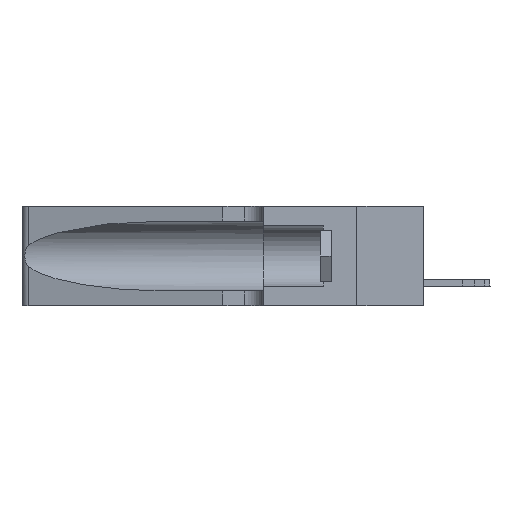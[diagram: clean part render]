
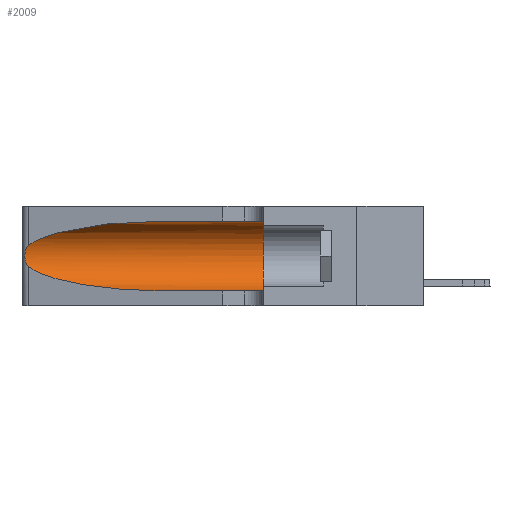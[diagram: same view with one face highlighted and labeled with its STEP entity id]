
A CAD part, left-side view. The second image highlights one B-rep face of the part: STEP entity #2009.
In plain terms, the highlighted cylindrical face has radius 3.308 mm (diameter 6.617 mm), a partial arc.
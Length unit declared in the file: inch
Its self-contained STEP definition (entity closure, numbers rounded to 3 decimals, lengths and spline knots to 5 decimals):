
#118 = VECTOR ( 'NONE', #12408, 39.37008 ) ;
#494 = CARTESIAN_POINT ( 'NONE',  ( 0.26075, 1.23896, 0.19203 ) ) ;
#770 = DIRECTION ( 'NONE',  ( 0., -1., 0. ) ) ;
#2009 = ADVANCED_FACE ( 'NONE', ( #16405 ), #30683, .F. ) ;
#2589 = CARTESIAN_POINT ( 'NONE',  ( 0.25856, 1.23593, 0.16098 ) ) ;
#2750 = CARTESIAN_POINT ( 'NONE',  ( 0.1305, 0.35, 0.31525 ) ) ;
#2858 = VERTEX_POINT ( 'NONE', #18748 ) ;
#3117 = DIRECTION ( 'NONE',  ( 0., 1., 0. ) ) ;
#3706 = EDGE_CURVE ( 'NONE', #29755, #21667, #17441, .T. ) ;
#3965 = EDGE_CURVE ( 'NONE', #21319, #2858, #20036, .T. ) ;
#4475 = CARTESIAN_POINT ( 'NONE',  ( 0.25487, 1.22718, 0.14631 ) ) ;
#4865 = AXIS2_PLACEMENT_3D ( 'NONE', #10769, #3117, #20255 ) ;
#5168 = CARTESIAN_POINT ( 'NONE',  ( 0.1305, 1.61858, 0.05475 ) ) ;
#5680 = CARTESIAN_POINT ( 'NONE',  ( 0.26075, 1.23896, 0.178 ) ) ;
#6440 = CARTESIAN_POINT ( 'NONE',  ( 0.1305, 0.72297, 0.31525 ) ) ;
#7777 = ORIENTED_EDGE ( 'NONE', *, *, #3965, .T. ) ;
#7809 =( BOUNDED_CURVE ( )  B_SPLINE_CURVE ( 3, ( #8480, #8130, #25208, #23164 ),
 .UNSPECIFIED., .F., .F. ) 
 B_SPLINE_CURVE_WITH_KNOTS ( ( 4, 4 ),
 ( 3.44316, 4.71239 ),
 .UNSPECIFIED. ) 
 CURVE ( )  GEOMETRIC_REPRESENTATION_ITEM ( )  RATIONAL_B_SPLINE_CURVE ( ( 1., 0.87, 0.87, 1. ) ) 
 REPRESENTATION_ITEM ( '' )  );
#7892 = CARTESIAN_POINT ( 'NONE',  ( 0.25787, 1.23484, 0.2124 ) ) ;
#8130 = CARTESIAN_POINT ( 'NONE',  ( 0.2373, 1.15595, 0.08982 ) ) ;
#8480 = CARTESIAN_POINT ( 'NONE',  ( 0.25487, 1.22718, 0.14631 ) ) ;
#9370 = ORIENTED_EDGE ( 'NONE', *, *, #3706, .T. ) ;
#9508 = EDGE_CURVE ( 'NONE', #17368, #21319, #7809, .T. ) ;
#10717 = CARTESIAN_POINT ( 'NONE',  ( 0.1305, 0.72297, 0.05475 ) ) ;
#10769 = CARTESIAN_POINT ( 'NONE',  ( 0.1305, 0.35, 0.185 ) ) ;
#10788 = AXIS2_PLACEMENT_3D ( 'NONE', #11399, #20803, #11186 ) ;
#11186 = DIRECTION ( 'NONE',  ( 0., 0., -1. ) ) ;
#11399 = CARTESIAN_POINT ( 'NONE',  ( 0.1305, 1.61858, 0.185 ) ) ;
#11884 = CARTESIAN_POINT ( 'NONE',  ( 0.1305, 1.61858, 0.31525 ) ) ;
#12408 = DIRECTION ( 'NONE',  ( 0., -1., 0. ) ) ;
#12956 = CARTESIAN_POINT ( 'NONE',  ( 0.25487, 1.22718, 0.22369 ) ) ;
#13177 = CIRCLE ( 'NONE', #4865, 0.13025 ) ;
#13243 = VERTEX_POINT ( 'NONE', #2750 ) ;
#15145 = CARTESIAN_POINT ( 'NONE',  ( 0.25854, 1.2359, 0.20912 ) ) ;
#16405 = FACE_OUTER_BOUND ( 'NONE', #19440, .T. ) ;
#16658 = EDGE_CURVE ( 'NONE', #21667, #17368, #19277, .T. ) ;
#16843 = CARTESIAN_POINT ( 'NONE',  ( 0.25487, 1.22718, 0.22369 ) ) ;
#17368 = VERTEX_POINT ( 'NONE', #4475 ) ;
#17374 = CARTESIAN_POINT ( 'NONE',  ( 0.25639, 1.23186, 0.15144 ) ) ;
#17441 =( BOUNDED_CURVE ( )  B_SPLINE_CURVE ( 3, ( #26740, #21963, #24543, #12956 ),
 .UNSPECIFIED., .F., .T. ) 
 B_SPLINE_CURVE_WITH_KNOTS ( ( 4, 4 ),
 ( 1.5708, 2.84003 ),
 .UNSPECIFIED. ) 
 CURVE ( )  GEOMETRIC_REPRESENTATION_ITEM ( )  RATIONAL_B_SPLINE_CURVE ( ( 1., 0.87, 0.87, 1. ) ) 
 REPRESENTATION_ITEM ( '' )  );
#17477 = EDGE_CURVE ( 'NONE', #29755, #13243, #30310, .T. ) ;
#17902 = CARTESIAN_POINT ( 'NONE',  ( 0.26018, 1.23835, 0.19895 ) ) ;
#18383 = EDGE_CURVE ( 'NONE', #13243, #2858, #13177, .T. ) ;
#18748 = CARTESIAN_POINT ( 'NONE',  ( 0.1305, 0.35, 0.05475 ) ) ;
#19277 = B_SPLINE_CURVE_WITH_KNOTS ( 'NONE', 3,
 ( #16843, #19337, #24567, #7892, #15145, #17902, #494, #5680, #25304, #2589, #22122, #17374, #22222, #29796 ),
 .UNSPECIFIED., .F., .F.,
 ( 4, 2, 2, 2, 2, 2, 4 ),
 ( 0., 0.00027, 0.00053, 0.00107, 0.0016, 0.00187, 0.00214 ),
 .UNSPECIFIED. ) ;
#19337 = CARTESIAN_POINT ( 'NONE',  ( 0.25555, 1.22994, 0.2215 ) ) ;
#19440 = EDGE_LOOP ( 'NONE', ( #9370, #25474, #23639, #7777, #22186, #31617 ) ) ;
#20036 = LINE ( 'NONE', #5168, #118 ) ;
#20255 = DIRECTION ( 'NONE',  ( 0., 0., 1. ) ) ;
#20803 = DIRECTION ( 'NONE',  ( 0., -1., 0. ) ) ;
#21014 = CARTESIAN_POINT ( 'NONE',  ( 0.25487, 1.22718, 0.22369 ) ) ;
#21319 = VERTEX_POINT ( 'NONE', #10717 ) ;
#21667 = VERTEX_POINT ( 'NONE', #21014 ) ;
#21963 = CARTESIAN_POINT ( 'NONE',  ( 0.18966, 0.96281, 0.31525 ) ) ;
#22122 = CARTESIAN_POINT ( 'NONE',  ( 0.25789, 1.23486, 0.15765 ) ) ;
#22186 = ORIENTED_EDGE ( 'NONE', *, *, #18383, .F. ) ;
#22222 = CARTESIAN_POINT ( 'NONE',  ( 0.25555, 1.22993, 0.14849 ) ) ;
#23164 = CARTESIAN_POINT ( 'NONE',  ( 0.1305, 0.72297, 0.05475 ) ) ;
#23639 = ORIENTED_EDGE ( 'NONE', *, *, #9508, .T. ) ;
#24543 = CARTESIAN_POINT ( 'NONE',  ( 0.2373, 1.15595, 0.28018 ) ) ;
#24567 = CARTESIAN_POINT ( 'NONE',  ( 0.25639, 1.23184, 0.21858 ) ) ;
#25208 = CARTESIAN_POINT ( 'NONE',  ( 0.18966, 0.96281, 0.05475 ) ) ;
#25304 = CARTESIAN_POINT ( 'NONE',  ( 0.26017, 1.23833, 0.17102 ) ) ;
#25474 = ORIENTED_EDGE ( 'NONE', *, *, #16658, .T. ) ;
#26740 = CARTESIAN_POINT ( 'NONE',  ( 0.1305, 0.72297, 0.31525 ) ) ;
#28775 = VECTOR ( 'NONE', #770, 39.37008 ) ;
#29755 = VERTEX_POINT ( 'NONE', #6440 ) ;
#29796 = CARTESIAN_POINT ( 'NONE',  ( 0.25487, 1.22718, 0.14631 ) ) ;
#30310 = LINE ( 'NONE', #11884, #28775 ) ;
#30683 = CYLINDRICAL_SURFACE ( 'NONE', #10788, 0.13025 ) ;
#31617 = ORIENTED_EDGE ( 'NONE', *, *, #17477, .F. ) ;
